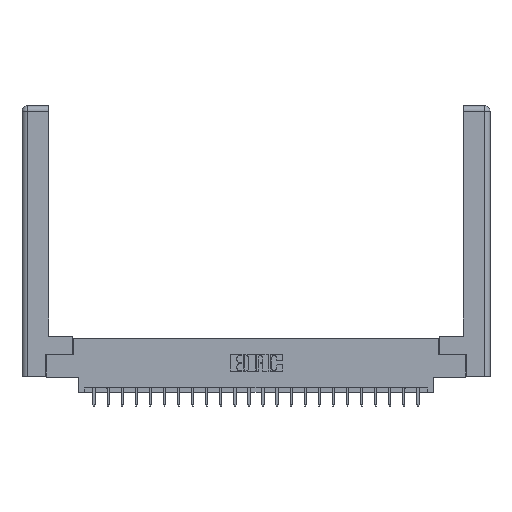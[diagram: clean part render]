
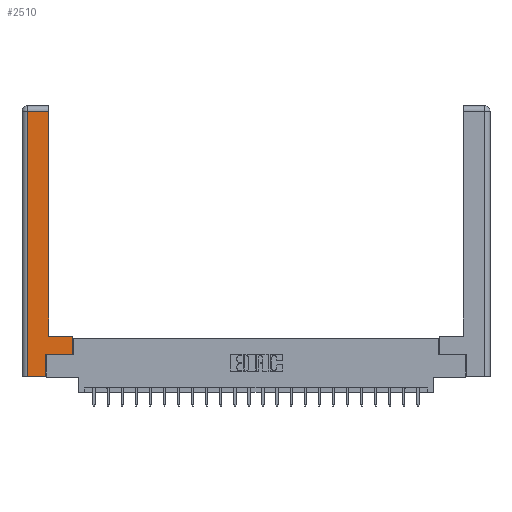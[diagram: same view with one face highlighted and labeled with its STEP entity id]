
A CAD part, top view. The second image highlights one B-rep face of the part: STEP entity #2510.
In plain terms, the highlighted planar face has unit normal (0, 0, 1).
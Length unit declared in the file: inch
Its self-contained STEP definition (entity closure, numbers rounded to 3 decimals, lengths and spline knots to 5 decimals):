
#18 = DIRECTION ( 'NONE',  ( 0., 1., 0. ) ) ;
#333 = VERTEX_POINT ( 'NONE', #13758 ) ;
#608 = VERTEX_POINT ( 'NONE', #7316 ) ;
#752 = CARTESIAN_POINT ( 'NONE',  ( 0.565, 0.45, 0. ) ) ;
#922 = EDGE_CURVE ( 'NONE', #333, #16753, #21243, .T. ) ;
#1340 = ORIENTED_EDGE ( 'NONE', *, *, #14489, .T. ) ;
#1868 = DIRECTION ( 'NONE',  ( 0., -1., 0. ) ) ;
#2198 = CARTESIAN_POINT ( 'NONE',  ( 0.0615, 2.94, 0. ) ) ;
#2415 = DIRECTION ( 'NONE',  ( 0., 0., -1. ) ) ;
#2510 = ADVANCED_FACE ( 'NONE', ( #20878 ), #15374, .F. ) ;
#2546 = CARTESIAN_POINT ( 'NONE',  ( 0.295, 2.94, 0. ) ) ;
#2648 = VERTEX_POINT ( 'NONE', #7581 ) ;
#3143 = DIRECTION ( 'NONE',  ( -1., 0., 0. ) ) ;
#3443 = LINE ( 'NONE', #4753, #4295 ) ;
#3655 = LINE ( 'NONE', #7209, #14828 ) ;
#4295 = VECTOR ( 'NONE', #3143, 39.37008 ) ;
#4481 = DIRECTION ( 'NONE',  ( -1., 0., 0. ) ) ;
#4555 = DIRECTION ( 'NONE',  ( -1., 0., 0. ) ) ;
#4753 = CARTESIAN_POINT ( 'NONE',  ( 0.295, 0.45, 0. ) ) ;
#5400 = LINE ( 'NONE', #16415, #6830 ) ;
#5713 = LINE ( 'NONE', #12075, #12298 ) ;
#6427 = DIRECTION ( 'NONE',  ( 0., 1., 0. ) ) ;
#6441 = AXIS2_PLACEMENT_3D ( 'NONE', #19136, #2415, #4481 ) ;
#6642 = VERTEX_POINT ( 'NONE', #2198 ) ;
#6830 = VECTOR ( 'NONE', #1868, 39.37008 ) ;
#6940 = ORIENTED_EDGE ( 'NONE', *, *, #15142, .T. ) ;
#7140 = ORIENTED_EDGE ( 'NONE', *, *, #20379, .T. ) ;
#7209 = CARTESIAN_POINT ( 'NONE',  ( 0.295, 3., 0. ) ) ;
#7316 = CARTESIAN_POINT ( 'NONE',  ( 0.565, 0.245, 0. ) ) ;
#7581 = CARTESIAN_POINT ( 'NONE',  ( 0.295, 0.45, 0. ) ) ;
#8034 = VERTEX_POINT ( 'NONE', #2546 ) ;
#8644 = ORIENTED_EDGE ( 'NONE', *, *, #21786, .T. ) ;
#9198 = VECTOR ( 'NONE', #6427, 39.37008 ) ;
#9291 = LINE ( 'NONE', #752, #12153 ) ;
#9330 = VERTEX_POINT ( 'NONE', #22695 ) ;
#10276 = LINE ( 'NONE', #18223, #20875 ) ;
#11796 = CARTESIAN_POINT ( 'NONE',  ( 0.265, 0.245, 0. ) ) ;
#11945 = DIRECTION ( 'NONE',  ( 0., 1., 0. ) ) ;
#12075 = CARTESIAN_POINT ( 'NONE',  ( 0.0615, 2.94, 0. ) ) ;
#12153 = VECTOR ( 'NONE', #11945, 39.37008 ) ;
#12298 = VECTOR ( 'NONE', #4555, 39.37008 ) ;
#13538 = DIRECTION ( 'NONE',  ( 1., 0., 0. ) ) ;
#13758 = CARTESIAN_POINT ( 'NONE',  ( 0.265, 0., 0. ) ) ;
#14335 = EDGE_CURVE ( 'NONE', #6642, #9330, #5400, .T. ) ;
#14489 = EDGE_CURVE ( 'NONE', #9330, #333, #21160, .T. ) ;
#14748 = CARTESIAN_POINT ( 'NONE',  ( 0.265, 0.245, 0. ) ) ;
#14828 = VECTOR ( 'NONE', #18, 39.37008 ) ;
#15142 = EDGE_CURVE ( 'NONE', #2648, #8034, #3655, .T. ) ;
#15374 = PLANE ( 'NONE',  #6441 ) ;
#15674 = ORIENTED_EDGE ( 'NONE', *, *, #922, .T. ) ;
#16216 = ORIENTED_EDGE ( 'NONE', *, *, #18557, .T. ) ;
#16415 = CARTESIAN_POINT ( 'NONE',  ( 0.0615, 0., 0. ) ) ;
#16454 = DIRECTION ( 'NONE',  ( 1., 0., 0. ) ) ;
#16753 = VERTEX_POINT ( 'NONE', #14748 ) ;
#17322 = ORIENTED_EDGE ( 'NONE', *, *, #14335, .T. ) ;
#18223 = CARTESIAN_POINT ( 'NONE',  ( 0.565, 0.245, 0. ) ) ;
#18330 = CARTESIAN_POINT ( 'NONE',  ( 0.565, 0.45, 0. ) ) ;
#18557 = EDGE_CURVE ( 'NONE', #608, #21528, #9291, .T. ) ;
#19136 = CARTESIAN_POINT ( 'NONE',  ( 0., 0., 0. ) ) ;
#19154 = VECTOR ( 'NONE', #13538, 39.37008 ) ;
#20379 = EDGE_CURVE ( 'NONE', #21528, #2648, #3443, .T. ) ;
#20669 = ORIENTED_EDGE ( 'NONE', *, *, #22233, .T. ) ;
#20875 = VECTOR ( 'NONE', #16454, 39.37008 ) ;
#20878 = FACE_OUTER_BOUND ( 'NONE', #22908, .T. ) ;
#21160 = LINE ( 'NONE', #22690, #19154 ) ;
#21243 = LINE ( 'NONE', #11796, #9198 ) ;
#21528 = VERTEX_POINT ( 'NONE', #18330 ) ;
#21786 = EDGE_CURVE ( 'NONE', #8034, #6642, #5713, .T. ) ;
#22233 = EDGE_CURVE ( 'NONE', #16753, #608, #10276, .T. ) ;
#22690 = CARTESIAN_POINT ( 'NONE',  ( 0.265, 0., 0. ) ) ;
#22695 = CARTESIAN_POINT ( 'NONE',  ( 0.0615, 0., 0. ) ) ;
#22908 = EDGE_LOOP ( 'NONE', ( #6940, #8644, #17322, #1340, #15674, #20669, #16216, #7140 ) ) ;
